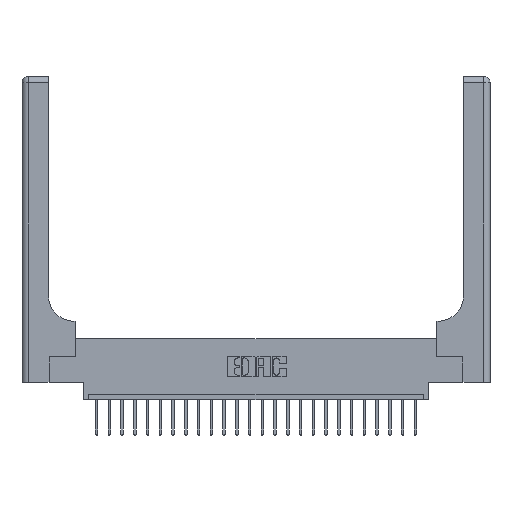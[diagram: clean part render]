
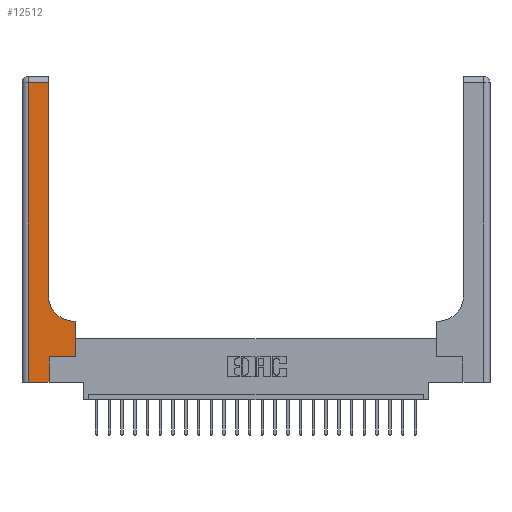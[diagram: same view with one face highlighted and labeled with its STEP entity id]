
A CAD part, top view. The second image highlights one B-rep face of the part: STEP entity #12512.
In plain terms, the highlighted planar face has unit normal (0, 0, 1).
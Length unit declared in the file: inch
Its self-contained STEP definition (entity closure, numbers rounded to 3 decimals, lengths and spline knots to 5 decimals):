
#465 = CIRCLE ( 'NONE', #19895, 0.25 ) ;
#504 = ORIENTED_EDGE ( 'NONE', *, *, #20354, .T. ) ;
#1091 = LINE ( 'NONE', #11917, #9900 ) ;
#1194 = ORIENTED_EDGE ( 'NONE', *, *, #16863, .T. ) ;
#1368 = CARTESIAN_POINT ( 'NONE',  ( 0.51, 0.85, 0.37 ) ) ;
#1552 = EDGE_CURVE ( 'NONE', #13845, #17410, #21866, .T. ) ;
#2057 = VECTOR ( 'NONE', #12286, 39.37008 ) ;
#2179 = CARTESIAN_POINT ( 'NONE',  ( 0.528, 0.25, 0.37 ) ) ;
#2218 = VECTOR ( 'NONE', #13639, 39.37008 ) ;
#2478 = LINE ( 'NONE', #21333, #4751 ) ;
#2533 = PLANE ( 'NONE',  #9373 ) ;
#2851 = CARTESIAN_POINT ( 'NONE',  ( 0.265, 0.25, 0.37 ) ) ;
#3105 = EDGE_CURVE ( 'NONE', #19346, #19560, #2478, .T. ) ;
#3173 = EDGE_CURVE ( 'NONE', #19560, #23913, #465, .T. ) ;
#3609 = VECTOR ( 'NONE', #5202, 39.37008 ) ;
#3827 = ORIENTED_EDGE ( 'NONE', *, *, #1552, .T. ) ;
#4258 = DIRECTION ( 'NONE',  ( -1., 0., 0. ) ) ;
#4751 = VECTOR ( 'NONE', #12075, 39.37008 ) ;
#4827 = ORIENTED_EDGE ( 'NONE', *, *, #13137, .T. ) ;
#4875 = CARTESIAN_POINT ( 'NONE',  ( 0.265, 0., 0.37 ) ) ;
#4970 = CARTESIAN_POINT ( 'NONE',  ( 0.26, 2.94, 0.37 ) ) ;
#5202 = DIRECTION ( 'NONE',  ( 0., -1., 0. ) ) ;
#6187 = DIRECTION ( 'NONE',  ( 0., 0., -1. ) ) ;
#6229 = CARTESIAN_POINT ( 'NONE',  ( 0.528, 0.25, 0.37 ) ) ;
#6804 = DIRECTION ( 'NONE',  ( -1., 0., 0. ) ) ;
#7132 = CARTESIAN_POINT ( 'NONE',  ( 0.06, 0., 0.37 ) ) ;
#7514 = ORIENTED_EDGE ( 'NONE', *, *, #15902, .T. ) ;
#8507 = LINE ( 'NONE', #12162, #2057 ) ;
#8821 = CARTESIAN_POINT ( 'NONE',  ( 0.06, 3., 0.37 ) ) ;
#9007 = ORIENTED_EDGE ( 'NONE', *, *, #3105, .T. ) ;
#9013 = CARTESIAN_POINT ( 'NONE',  ( 0.528, 0.6, 0.37 ) ) ;
#9373 = AXIS2_PLACEMENT_3D ( 'NONE', #20917, #6187, #4258 ) ;
#9900 = VECTOR ( 'NONE', #6804, 39.37008 ) ;
#10492 = DIRECTION ( 'NONE',  ( 0., 0., -1. ) ) ;
#10902 = LINE ( 'NONE', #8821, #3609 ) ;
#10914 = CARTESIAN_POINT ( 'NONE',  ( 0.265, 0.25, 0.37 ) ) ;
#11116 = ORIENTED_EDGE ( 'NONE', *, *, #20180, .T. ) ;
#11224 = CARTESIAN_POINT ( 'NONE',  ( 0.26, 0.85, 0.37 ) ) ;
#11376 = VERTEX_POINT ( 'NONE', #12258 ) ;
#11917 = CARTESIAN_POINT ( 'NONE',  ( 0., 2.94, 0.37 ) ) ;
#12075 = DIRECTION ( 'NONE',  ( -1., 0., 0. ) ) ;
#12162 = CARTESIAN_POINT ( 'NONE',  ( 0., 0., 0.37 ) ) ;
#12258 = CARTESIAN_POINT ( 'NONE',  ( 0.06, 2.94, 0.37 ) ) ;
#12286 = DIRECTION ( 'NONE',  ( 1., 0., 0. ) ) ;
#12512 = ADVANCED_FACE ( 'NONE', ( #16815 ), #2533, .F. ) ;
#12633 = EDGE_LOOP ( 'NONE', ( #504, #7514, #4827, #18232, #1194, #3827, #11116, #9007, #21642 ) ) ;
#13137 = EDGE_CURVE ( 'NONE', #11376, #23452, #10902, .T. ) ;
#13639 = DIRECTION ( 'NONE',  ( 0., 1., 0. ) ) ;
#13667 = EDGE_CURVE ( 'NONE', #23452, #14748, #8507, .T. ) ;
#13764 = LINE ( 'NONE', #21196, #22439 ) ;
#13845 = VERTEX_POINT ( 'NONE', #2851 ) ;
#14748 = VERTEX_POINT ( 'NONE', #4875 ) ;
#15555 = CARTESIAN_POINT ( 'NONE',  ( 0.51, 0.6, 0.37 ) ) ;
#15902 = EDGE_CURVE ( 'NONE', #21282, #11376, #1091, .T. ) ;
#16815 = FACE_OUTER_BOUND ( 'NONE', #12633, .T. ) ;
#16863 = EDGE_CURVE ( 'NONE', #14748, #13845, #17947, .T. ) ;
#17069 = LINE ( 'NONE', #6229, #2218 ) ;
#17397 = VECTOR ( 'NONE', #20284, 39.37008 ) ;
#17410 = VERTEX_POINT ( 'NONE', #2179 ) ;
#17537 = DIRECTION ( 'NONE',  ( 0., 1., 0. ) ) ;
#17947 = LINE ( 'NONE', #23417, #21977 ) ;
#18232 = ORIENTED_EDGE ( 'NONE', *, *, #13667, .T. ) ;
#19346 = VERTEX_POINT ( 'NONE', #9013 ) ;
#19560 = VERTEX_POINT ( 'NONE', #15555 ) ;
#19770 = DIRECTION ( 'NONE',  ( 0., 1., 0. ) ) ;
#19872 = DIRECTION ( 'NONE',  ( 1., 0., 0. ) ) ;
#19895 = AXIS2_PLACEMENT_3D ( 'NONE', #1368, #10492, #19872 ) ;
#20180 = EDGE_CURVE ( 'NONE', #17410, #19346, #17069, .T. ) ;
#20284 = DIRECTION ( 'NONE',  ( 1., 0., 0. ) ) ;
#20354 = EDGE_CURVE ( 'NONE', #23913, #21282, #13764, .T. ) ;
#20917 = CARTESIAN_POINT ( 'NONE',  ( 0., 3., 0.37 ) ) ;
#21196 = CARTESIAN_POINT ( 'NONE',  ( 0.26, 3., 0.37 ) ) ;
#21282 = VERTEX_POINT ( 'NONE', #4970 ) ;
#21333 = CARTESIAN_POINT ( 'NONE',  ( 0.26, 0.6, 0.37 ) ) ;
#21642 = ORIENTED_EDGE ( 'NONE', *, *, #3173, .T. ) ;
#21866 = LINE ( 'NONE', #10914, #17397 ) ;
#21977 = VECTOR ( 'NONE', #19770, 39.37008 ) ;
#22439 = VECTOR ( 'NONE', #17537, 39.37008 ) ;
#23417 = CARTESIAN_POINT ( 'NONE',  ( 0.265, 0., 0.37 ) ) ;
#23452 = VERTEX_POINT ( 'NONE', #7132 ) ;
#23913 = VERTEX_POINT ( 'NONE', #11224 ) ;
